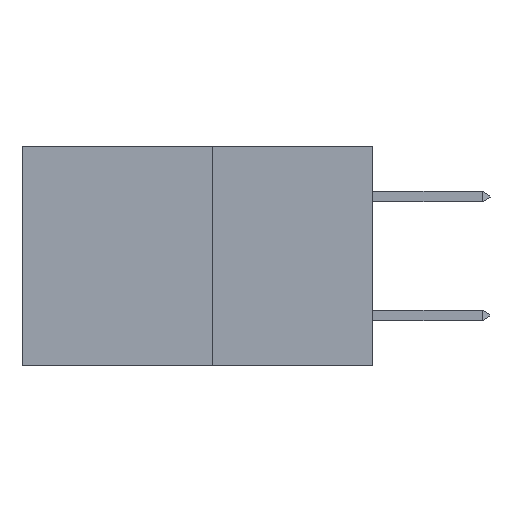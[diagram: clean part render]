
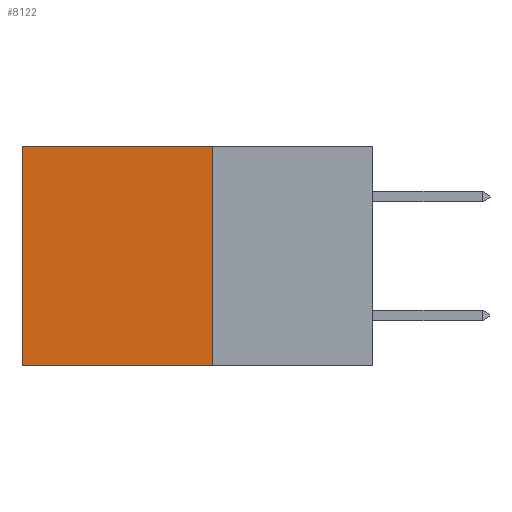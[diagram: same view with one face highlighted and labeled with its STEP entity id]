
A CAD part, left-side view. The second image highlights one B-rep face of the part: STEP entity #8122.
In plain terms, the highlighted planar face has unit normal (-1, 0, 0).
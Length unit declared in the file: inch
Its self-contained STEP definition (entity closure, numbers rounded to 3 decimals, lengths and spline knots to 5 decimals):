
#174 = EDGE_LOOP ( 'NONE', ( #5611, #3193, #10183, #8851 ) ) ;
#183 = VERTEX_POINT ( 'NONE', #4659 ) ;
#597 = DIRECTION ( 'NONE',  ( 0., 1., 0. ) ) ;
#783 = LINE ( 'NONE', #1753, #3297 ) ;
#1310 = EDGE_CURVE ( 'NONE', #8746, #7547, #6411, .T. ) ;
#1348 = DIRECTION ( 'NONE',  ( 0., 0., -1. ) ) ;
#1703 = EDGE_CURVE ( 'NONE', #183, #8746, #4883, .T. ) ;
#1752 = LINE ( 'NONE', #9582, #10810 ) ;
#1753 = CARTESIAN_POINT ( 'NONE',  ( 0.277, 0.27, 0. ) ) ;
#2065 = EDGE_CURVE ( 'NONE', #7370, #7547, #1752, .T. ) ;
#2581 = FACE_OUTER_BOUND ( 'NONE', #174, .T. ) ;
#2776 = PLANE ( 'NONE',  #10879 ) ;
#3193 = ORIENTED_EDGE ( 'NONE', *, *, #1310, .F. ) ;
#3297 = VECTOR ( 'NONE', #597, 39.37008 ) ;
#3440 = EDGE_CURVE ( 'NONE', #183, #7370, #783, .T. ) ;
#4248 = CARTESIAN_POINT ( 'NONE',  ( 0.277, 0.27, -0.37 ) ) ;
#4588 = CARTESIAN_POINT ( 'NONE',  ( 0.277, 0.59, -0.37 ) ) ;
#4644 = DIRECTION ( 'NONE',  ( 0., 0., -1. ) ) ;
#4659 = CARTESIAN_POINT ( 'NONE',  ( 0.277, 0.27, 0. ) ) ;
#4821 = CARTESIAN_POINT ( 'NONE',  ( 0.277, 0.27, -0.37 ) ) ;
#4883 = LINE ( 'NONE', #4248, #9230 ) ;
#5611 = ORIENTED_EDGE ( 'NONE', *, *, #2065, .T. ) ;
#5623 = DIRECTION ( 'NONE',  ( 0., 0., -1. ) ) ;
#6139 = VECTOR ( 'NONE', #7911, 39.37008 ) ;
#6411 = LINE ( 'NONE', #4821, #6139 ) ;
#6977 = CARTESIAN_POINT ( 'NONE',  ( 0.277, 0.59, 0. ) ) ;
#7214 = CARTESIAN_POINT ( 'NONE',  ( 0.277, 0.27, -0.37 ) ) ;
#7370 = VERTEX_POINT ( 'NONE', #6977 ) ;
#7547 = VERTEX_POINT ( 'NONE', #4588 ) ;
#7911 = DIRECTION ( 'NONE',  ( 0., 1., 0. ) ) ;
#8122 = ADVANCED_FACE ( 'NONE', ( #2581 ), #2776, .F. ) ;
#8746 = VERTEX_POINT ( 'NONE', #9003 ) ;
#8851 = ORIENTED_EDGE ( 'NONE', *, *, #3440, .T. ) ;
#9003 = CARTESIAN_POINT ( 'NONE',  ( 0.277, 0.27, -0.37 ) ) ;
#9230 = VECTOR ( 'NONE', #1348, 39.37008 ) ;
#9582 = CARTESIAN_POINT ( 'NONE',  ( 0.277, 0.59, -0.37 ) ) ;
#9836 = DIRECTION ( 'NONE',  ( 1., 0., 0. ) ) ;
#10183 = ORIENTED_EDGE ( 'NONE', *, *, #1703, .F. ) ;
#10810 = VECTOR ( 'NONE', #5623, 39.37008 ) ;
#10879 = AXIS2_PLACEMENT_3D ( 'NONE', #7214, #9836, #4644 ) ;
